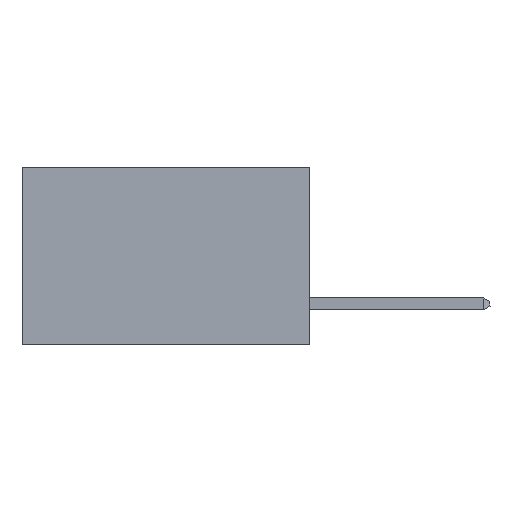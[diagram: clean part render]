
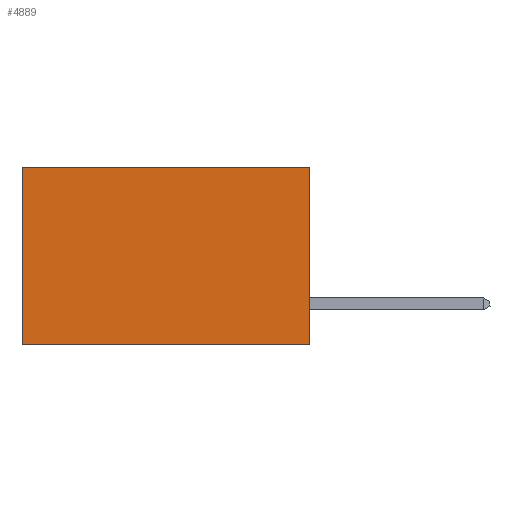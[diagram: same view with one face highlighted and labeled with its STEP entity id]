
A CAD part, left-side view. The second image highlights one B-rep face of the part: STEP entity #4889.
In plain terms, the highlighted planar face has unit normal (-1, 0, 0).
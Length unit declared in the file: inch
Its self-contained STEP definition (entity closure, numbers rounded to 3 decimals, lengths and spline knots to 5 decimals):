
#91 = DIRECTION ( 'NONE',  ( 0., 1., 0. ) ) ;
#560 = LINE ( 'NONE', #11292, #711 ) ;
#711 = VECTOR ( 'NONE', #91, 39.37008 ) ;
#736 = DIRECTION ( 'NONE',  ( 0., 1., 0. ) ) ;
#968 = CARTESIAN_POINT ( 'NONE',  ( 0.2875, 0., 0. ) ) ;
#1017 = VECTOR ( 'NONE', #11436, 39.37008 ) ;
#1525 = FACE_OUTER_BOUND ( 'NONE', #4721, .T. ) ;
#1887 = PLANE ( 'NONE',  #11386 ) ;
#1931 = EDGE_CURVE ( 'NONE', #8398, #4312, #2493, .T. ) ;
#2248 = VERTEX_POINT ( 'NONE', #11172 ) ;
#2493 = LINE ( 'NONE', #3016, #1017 ) ;
#2915 = ORIENTED_EDGE ( 'NONE', *, *, #5137, .T. ) ;
#3016 = CARTESIAN_POINT ( 'NONE',  ( 0.2875, 0., 0. ) ) ;
#3021 = CARTESIAN_POINT ( 'NONE',  ( 0.2875, 0., -0.37 ) ) ;
#3460 = CARTESIAN_POINT ( 'NONE',  ( 0.2875, 0., 0. ) ) ;
#3542 = CARTESIAN_POINT ( 'NONE',  ( 0.2875, 0., 0. ) ) ;
#3796 = LINE ( 'NONE', #4306, #6431 ) ;
#4306 = CARTESIAN_POINT ( 'NONE',  ( 0.2875, 0.6, 0. ) ) ;
#4312 = VERTEX_POINT ( 'NONE', #3021 ) ;
#4721 = EDGE_LOOP ( 'NONE', ( #9591, #7064, #8410, #2915 ) ) ;
#4889 = ADVANCED_FACE ( 'NONE', ( #1525 ), #1887, .F. ) ;
#5137 = EDGE_CURVE ( 'NONE', #8398, #11006, #10197, .T. ) ;
#5165 = DIRECTION ( 'NONE',  ( 0., 0., -1. ) ) ;
#6431 = VECTOR ( 'NONE', #5165, 39.37008 ) ;
#7064 = ORIENTED_EDGE ( 'NONE', *, *, #9835, .F. ) ;
#7543 = DIRECTION ( 'NONE',  ( 1., 0., 0. ) ) ;
#8398 = VERTEX_POINT ( 'NONE', #3460 ) ;
#8410 = ORIENTED_EDGE ( 'NONE', *, *, #1931, .F. ) ;
#9460 = DIRECTION ( 'NONE',  ( 0., 0., -1. ) ) ;
#9591 = ORIENTED_EDGE ( 'NONE', *, *, #10941, .T. ) ;
#9619 = VECTOR ( 'NONE', #736, 39.37008 ) ;
#9835 = EDGE_CURVE ( 'NONE', #4312, #2248, #560, .T. ) ;
#9897 = CARTESIAN_POINT ( 'NONE',  ( 0.2875, 0.6, 0. ) ) ;
#10197 = LINE ( 'NONE', #3542, #9619 ) ;
#10941 = EDGE_CURVE ( 'NONE', #11006, #2248, #3796, .T. ) ;
#11006 = VERTEX_POINT ( 'NONE', #9897 ) ;
#11172 = CARTESIAN_POINT ( 'NONE',  ( 0.2875, 0.6, -0.37 ) ) ;
#11292 = CARTESIAN_POINT ( 'NONE',  ( 0.2875, 0., -0.37 ) ) ;
#11386 = AXIS2_PLACEMENT_3D ( 'NONE', #968, #7543, #9460 ) ;
#11436 = DIRECTION ( 'NONE',  ( 0., 0., -1. ) ) ;
